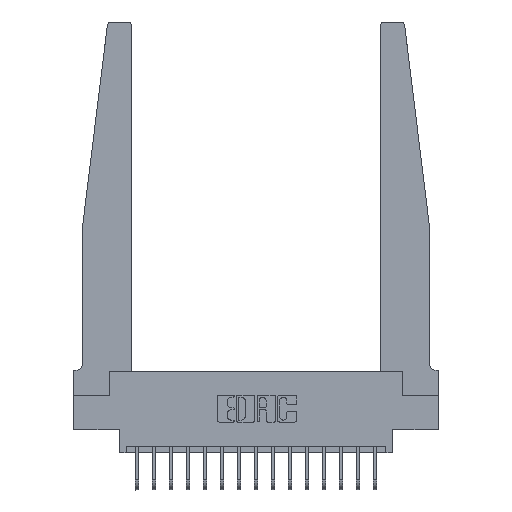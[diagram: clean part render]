
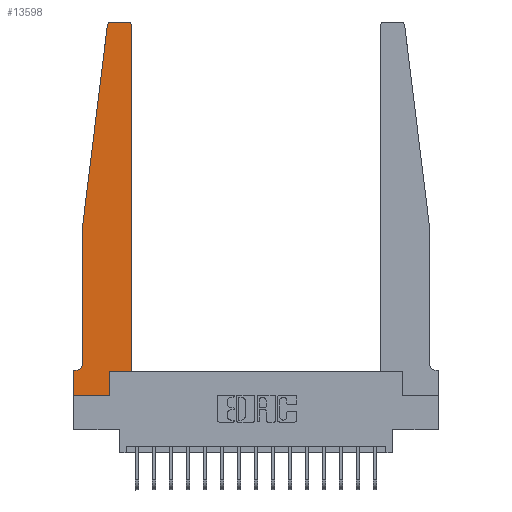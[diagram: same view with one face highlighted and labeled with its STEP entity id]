
A CAD part, top view. The second image highlights one B-rep face of the part: STEP entity #13598.
In plain terms, the highlighted planar face has unit normal (0, 0, 1).
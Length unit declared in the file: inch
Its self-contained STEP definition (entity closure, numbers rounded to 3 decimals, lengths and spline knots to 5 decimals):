
#208 = LINE ( 'NONE', #7355, #8529 ) ;
#224 = DIRECTION ( 'NONE',  ( -1., 0., 0. ) ) ;
#466 = ORIENTED_EDGE ( 'NONE', *, *, #13282, .T. ) ;
#711 = ORIENTED_EDGE ( 'NONE', *, *, #12557, .T. ) ;
#1036 = CIRCLE ( 'NONE', #8158, 0.03 ) ;
#1042 = ORIENTED_EDGE ( 'NONE', *, *, #10343, .T. ) ;
#1078 = VECTOR ( 'NONE', #14863, 39.37008 ) ;
#1269 = CARTESIAN_POINT ( 'NONE',  ( 0.2605, 0.18, 0.37 ) ) ;
#1321 = DIRECTION ( 'NONE',  ( 0., 0., -1. ) ) ;
#1556 = CARTESIAN_POINT ( 'NONE',  ( 0.27653, 2.72, 0.37 ) ) ;
#1672 = EDGE_CURVE ( 'NONE', #9268, #10576, #17776, .T. ) ;
#1710 = ORIENTED_EDGE ( 'NONE', *, *, #6483, .T. ) ;
#2028 = VERTEX_POINT ( 'NONE', #10439 ) ;
#2314 = ORIENTED_EDGE ( 'NONE', *, *, #9597, .T. ) ;
#2340 = LINE ( 'NONE', #8196, #1078 ) ;
#2634 = VERTEX_POINT ( 'NONE', #8611 ) ;
#2746 = CARTESIAN_POINT ( 'NONE',  ( 0.425, 2.72, 0.37 ) ) ;
#3150 = CARTESIAN_POINT ( 'NONE',  ( 0.065, 1.25, 0.37 ) ) ;
#3488 = PLANE ( 'NONE',  #15553 ) ;
#3557 = CARTESIAN_POINT ( 'NONE',  ( 0.065, 1.25, 0.37 ) ) ;
#3643 = LINE ( 'NONE', #3557, #8456 ) ;
#3814 = CARTESIAN_POINT ( 'NONE',  ( 0., 0.1875, 0.37 ) ) ;
#3887 = EDGE_LOOP ( 'NONE', ( #2314, #466, #9732, #18276, #711, #1710, #9688, #13232, #1042, #12735, #17951, #6049 ) ) ;
#4162 = VECTOR ( 'NONE', #224, 39.37008 ) ;
#4876 = CARTESIAN_POINT ( 'NONE',  ( 0.425, 0.18, 0.37 ) ) ;
#4910 = LINE ( 'NONE', #1269, #12402 ) ;
#4936 = DIRECTION ( 'NONE',  ( 0., 1., 0. ) ) ;
#5000 = VERTEX_POINT ( 'NONE', #17162 ) ;
#5367 = EDGE_CURVE ( 'NONE', #13310, #14296, #1036, .T. ) ;
#6010 = DIRECTION ( 'NONE',  ( 0., 0., 1. ) ) ;
#6049 = ORIENTED_EDGE ( 'NONE', *, *, #5367, .T. ) ;
#6069 = AXIS2_PLACEMENT_3D ( 'NONE', #1556, #11398, #14166 ) ;
#6390 = DIRECTION ( 'NONE',  ( 0., 1., 0. ) ) ;
#6428 = CARTESIAN_POINT ( 'NONE',  ( 0.425, 0.18, 0.37 ) ) ;
#6483 = EDGE_CURVE ( 'NONE', #16185, #8483, #8932, .T. ) ;
#6613 = AXIS2_PLACEMENT_3D ( 'NONE', #14020, #1321, #15520 ) ;
#6747 = CARTESIAN_POINT ( 'NONE',  ( 0., 0., 0.37 ) ) ;
#6988 = VECTOR ( 'NONE', #14471, 39.37008 ) ;
#7172 = DIRECTION ( 'NONE',  ( 0., -1., 0. ) ) ;
#7355 = CARTESIAN_POINT ( 'NONE',  ( 0.065, 1.25, 0.37 ) ) ;
#7585 = VERTEX_POINT ( 'NONE', #3150 ) ;
#8064 = VERTEX_POINT ( 'NONE', #13182 ) ;
#8158 = AXIS2_PLACEMENT_3D ( 'NONE', #18283, #6010, #16044 ) ;
#8196 = CARTESIAN_POINT ( 'NONE',  ( 0., 0., 0.37 ) ) ;
#8456 = VECTOR ( 'NONE', #17852, 39.37008 ) ;
#8458 = VERTEX_POINT ( 'NONE', #16004 ) ;
#8483 = VERTEX_POINT ( 'NONE', #3814 ) ;
#8529 = VECTOR ( 'NONE', #7172, 39.37008 ) ;
#8611 = CARTESIAN_POINT ( 'NONE',  ( 0., 0., 0.37 ) ) ;
#8932 = LINE ( 'NONE', #16997, #6988 ) ;
#8953 = CARTESIAN_POINT ( 'NONE',  ( 0.395, 2.75, 0.37 ) ) ;
#9168 = CARTESIAN_POINT ( 'NONE',  ( 0., 0.1875, 0.37 ) ) ;
#9268 = VERTEX_POINT ( 'NONE', #17327 ) ;
#9597 = EDGE_CURVE ( 'NONE', #14296, #8458, #12682, .T. ) ;
#9688 = ORIENTED_EDGE ( 'NONE', *, *, #16091, .T. ) ;
#9732 = ORIENTED_EDGE ( 'NONE', *, *, #13985, .T. ) ;
#9761 = EDGE_CURVE ( 'NONE', #10576, #13310, #11736, .T. ) ;
#9863 = EDGE_CURVE ( 'NONE', #2634, #2028, #2340, .T. ) ;
#9987 = VECTOR ( 'NONE', #15941, 39.37008 ) ;
#10069 = CARTESIAN_POINT ( 'NONE',  ( 0.25, 2.75, 0.37 ) ) ;
#10343 = EDGE_CURVE ( 'NONE', #2028, #9268, #4910, .T. ) ;
#10439 = CARTESIAN_POINT ( 'NONE',  ( 0.2605, 0., 0.37 ) ) ;
#10576 = VERTEX_POINT ( 'NONE', #4876 ) ;
#10651 = VECTOR ( 'NONE', #17857, 39.37008 ) ;
#10829 = FACE_OUTER_BOUND ( 'NONE', #3887, .T. ) ;
#11398 = DIRECTION ( 'NONE',  ( 0., 0., 1. ) ) ;
#11736 = LINE ( 'NONE', #12012, #17819 ) ;
#12012 = CARTESIAN_POINT ( 'NONE',  ( 0.425, 0.18, 0.37 ) ) ;
#12047 = DIRECTION ( 'NONE',  ( 0., 0., 1. ) ) ;
#12402 = VECTOR ( 'NONE', #6390, 39.37008 ) ;
#12557 = EDGE_CURVE ( 'NONE', #8064, #16185, #15200, .T. ) ;
#12682 = LINE ( 'NONE', #10069, #4162 ) ;
#12735 = ORIENTED_EDGE ( 'NONE', *, *, #1672, .T. ) ;
#13182 = CARTESIAN_POINT ( 'NONE',  ( 0.065, 0.2375, 0.37 ) ) ;
#13232 = ORIENTED_EDGE ( 'NONE', *, *, #9863, .T. ) ;
#13282 = EDGE_CURVE ( 'NONE', #8458, #5000, #14637, .T. ) ;
#13310 = VERTEX_POINT ( 'NONE', #2746 ) ;
#13526 = DIRECTION ( 'NONE',  ( 1., 0., 0. ) ) ;
#13598 = ADVANCED_FACE ( 'NONE', ( #10829 ), #3488, .T. ) ;
#13812 = LINE ( 'NONE', #6747, #9987 ) ;
#13985 = EDGE_CURVE ( 'NONE', #5000, #7585, #3643, .T. ) ;
#14020 = CARTESIAN_POINT ( 'NONE',  ( 0.015, 0.2375, 0.37 ) ) ;
#14166 = DIRECTION ( 'NONE',  ( 1., 0., 0. ) ) ;
#14296 = VERTEX_POINT ( 'NONE', #8953 ) ;
#14471 = DIRECTION ( 'NONE',  ( -1., 0., 0. ) ) ;
#14637 = CIRCLE ( 'NONE', #6069, 0.03 ) ;
#14863 = DIRECTION ( 'NONE',  ( 1., 0., 0. ) ) ;
#15200 = CIRCLE ( 'NONE', #6613, 0.05 ) ;
#15520 = DIRECTION ( 'NONE',  ( -1., 0., 0. ) ) ;
#15553 = AXIS2_PLACEMENT_3D ( 'NONE', #9168, #12047, #13526 ) ;
#15676 = CARTESIAN_POINT ( 'NONE',  ( 0.015, 0.1875, 0.37 ) ) ;
#15941 = DIRECTION ( 'NONE',  ( 0., -1., 0. ) ) ;
#16004 = CARTESIAN_POINT ( 'NONE',  ( 0.27653, 2.75, 0.37 ) ) ;
#16044 = DIRECTION ( 'NONE',  ( 1., 0., 0. ) ) ;
#16091 = EDGE_CURVE ( 'NONE', #8483, #2634, #13812, .T. ) ;
#16185 = VERTEX_POINT ( 'NONE', #15676 ) ;
#16997 = CARTESIAN_POINT ( 'NONE',  ( 0.065, 0.1875, 0.37 ) ) ;
#17162 = CARTESIAN_POINT ( 'NONE',  ( 0.24675, 2.72367, 0.37 ) ) ;
#17327 = CARTESIAN_POINT ( 'NONE',  ( 0.2605, 0.18, 0.37 ) ) ;
#17776 = LINE ( 'NONE', #6428, #10651 ) ;
#17819 = VECTOR ( 'NONE', #4936, 39.37008 ) ;
#17852 = DIRECTION ( 'NONE',  ( -0.122, -0.992, 0. ) ) ;
#17857 = DIRECTION ( 'NONE',  ( 1., 0., 0. ) ) ;
#17938 = EDGE_CURVE ( 'NONE', #7585, #8064, #208, .T. ) ;
#17951 = ORIENTED_EDGE ( 'NONE', *, *, #9761, .T. ) ;
#18276 = ORIENTED_EDGE ( 'NONE', *, *, #17938, .T. ) ;
#18283 = CARTESIAN_POINT ( 'NONE',  ( 0.395, 2.72, 0.37 ) ) ;
